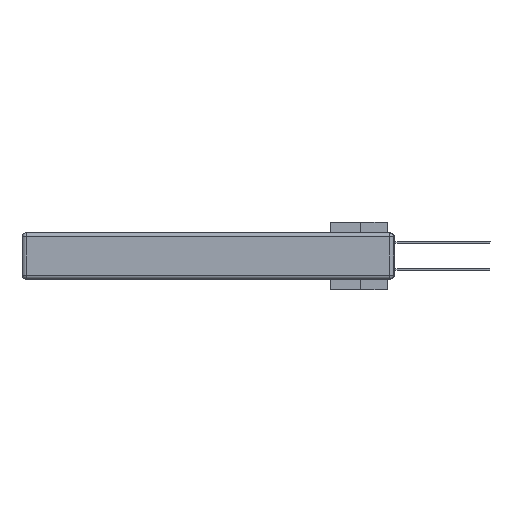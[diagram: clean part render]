
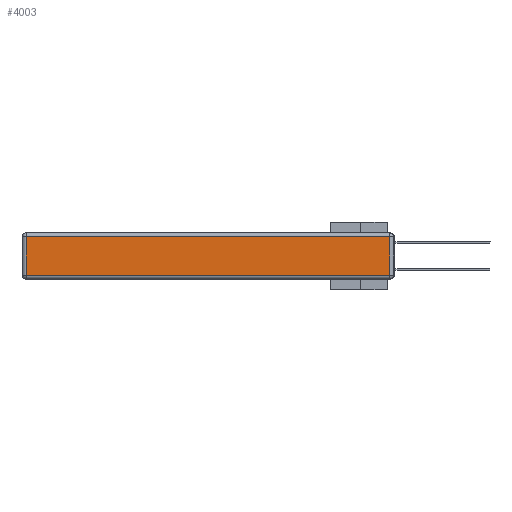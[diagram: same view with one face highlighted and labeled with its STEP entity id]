
A CAD part, left-side view. The second image highlights one B-rep face of the part: STEP entity #4003.
In plain terms, the highlighted planar face has unit normal (-1, 0, 0).
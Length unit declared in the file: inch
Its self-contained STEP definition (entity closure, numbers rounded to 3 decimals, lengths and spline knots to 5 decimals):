
#1323 = FACE_OUTER_BOUND ( 'NONE', #34036, .T. ) ;
#1589 = CARTESIAN_POINT ( 'NONE',  ( 0., 0.03, -0.313 ) ) ;
#2300 = VERTEX_POINT ( 'NONE', #1589 ) ;
#2899 = CARTESIAN_POINT ( 'NONE',  ( 0., 0.03, -0.343 ) ) ;
#4003 = ADVANCED_FACE ( 'NONE', ( #1323 ), #9361, .T. ) ;
#5978 = DIRECTION ( 'NONE',  ( 0., 0., 1. ) ) ;
#5982 = ORIENTED_EDGE ( 'NONE', *, *, #7073, .T. ) ;
#6695 = VERTEX_POINT ( 'NONE', #12764 ) ;
#7073 = EDGE_CURVE ( 'NONE', #6695, #12354, #29772, .T. ) ;
#7101 = ORIENTED_EDGE ( 'NONE', *, *, #10258, .T. ) ;
#8055 = CARTESIAN_POINT ( 'NONE',  ( 0., 0.03, -0.03 ) ) ;
#8091 = CARTESIAN_POINT ( 'NONE',  ( 0., 2.72, -0.313 ) ) ;
#9254 = VECTOR ( 'NONE', #18482, 39.37008 ) ;
#9361 = PLANE ( 'NONE',  #20674 ) ;
#9544 = CARTESIAN_POINT ( 'NONE',  ( 0., 0., -0.343 ) ) ;
#10010 = DIRECTION ( 'NONE',  ( 0., 1., 0. ) ) ;
#10258 = EDGE_CURVE ( 'NONE', #2300, #14013, #20707, .T. ) ;
#10723 = VECTOR ( 'NONE', #10010, 39.37008 ) ;
#12354 = VERTEX_POINT ( 'NONE', #8091 ) ;
#12764 = CARTESIAN_POINT ( 'NONE',  ( 0., 2.72, -0.03 ) ) ;
#14013 = VERTEX_POINT ( 'NONE', #8055 ) ;
#16924 = EDGE_CURVE ( 'NONE', #14013, #6695, #24575, .T. ) ;
#18482 = DIRECTION ( 'NONE',  ( 0., 0., -1. ) ) ;
#18550 = DIRECTION ( 'NONE',  ( -1., 0., 0. ) ) ;
#19356 = ORIENTED_EDGE ( 'NONE', *, *, #16924, .T. ) ;
#20483 = ORIENTED_EDGE ( 'NONE', *, *, #37570, .T. ) ;
#20674 = AXIS2_PLACEMENT_3D ( 'NONE', #9544, #18550, #35778 ) ;
#20707 = LINE ( 'NONE', #2899, #33823 ) ;
#22808 = CARTESIAN_POINT ( 'NONE',  ( 0., 0., -0.313 ) ) ;
#24575 = LINE ( 'NONE', #36252, #10723 ) ;
#25880 = DIRECTION ( 'NONE',  ( 0., -1., 0. ) ) ;
#29772 = LINE ( 'NONE', #30521, #9254 ) ;
#30521 = CARTESIAN_POINT ( 'NONE',  ( 0., 2.72, -0.343 ) ) ;
#33823 = VECTOR ( 'NONE', #5978, 39.37008 ) ;
#34036 = EDGE_LOOP ( 'NONE', ( #20483, #7101, #19356, #5982 ) ) ;
#34354 = VECTOR ( 'NONE', #25880, 39.37008 ) ;
#35778 = DIRECTION ( 'NONE',  ( 0., 0., 1. ) ) ;
#36252 = CARTESIAN_POINT ( 'NONE',  ( 0., 2.75, -0.03 ) ) ;
#37166 = LINE ( 'NONE', #22808, #34354 ) ;
#37570 = EDGE_CURVE ( 'NONE', #12354, #2300, #37166, .T. ) ;
